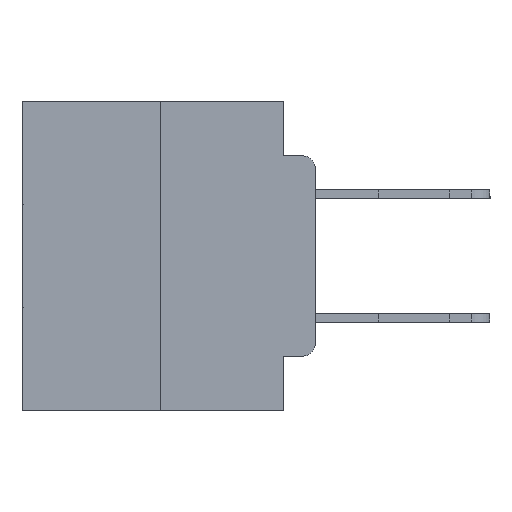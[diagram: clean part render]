
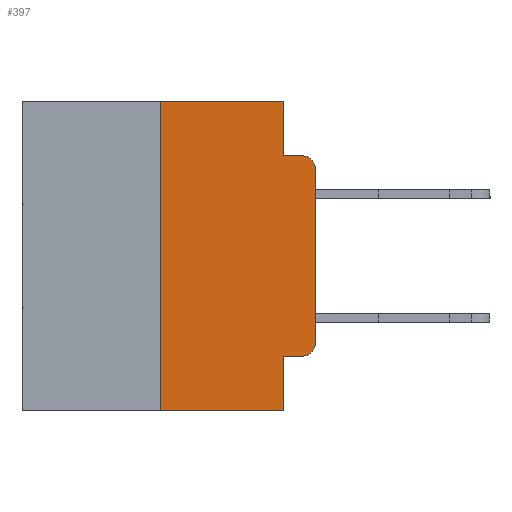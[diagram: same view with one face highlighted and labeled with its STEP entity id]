
A CAD part, left-side view. The second image highlights one B-rep face of the part: STEP entity #397.
In plain terms, the highlighted planar face has unit normal (-1, 0, 0).
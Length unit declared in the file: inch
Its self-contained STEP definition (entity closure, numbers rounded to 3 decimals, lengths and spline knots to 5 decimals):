
#229 = LINE ( 'NONE', #26358, #16529 ) ;
#397 = ADVANCED_FACE ( 'NONE', ( #26784 ), #27056, .F. ) ;
#853 = VERTEX_POINT ( 'NONE', #21630 ) ;
#1087 = VECTOR ( 'NONE', #23275, 39.37008 ) ;
#1859 = ORIENTED_EDGE ( 'NONE', *, *, #12511, .F. ) ;
#2058 = LINE ( 'NONE', #12790, #23794 ) ;
#2089 = CARTESIAN_POINT ( 'NONE',  ( 0., 0.051, 0. ) ) ;
#2174 = VERTEX_POINT ( 'NONE', #6560 ) ;
#2223 = ORIENTED_EDGE ( 'NONE', *, *, #10779, .T. ) ;
#2288 = LINE ( 'NONE', #14932, #2965 ) ;
#2649 = LINE ( 'NONE', #8467, #24348 ) ;
#2965 = VECTOR ( 'NONE', #25342, 39.37008 ) ;
#3467 = CARTESIAN_POINT ( 'NONE',  ( 0., 0.02, -0.1085 ) ) ;
#3753 = VECTOR ( 'NONE', #7286, 39.37008 ) ;
#4830 = CIRCLE ( 'NONE', #24839, 0.02 ) ;
#5434 = CARTESIAN_POINT ( 'NONE',  ( 0., 0., -0.1085 ) ) ;
#5666 = DIRECTION ( 'NONE',  ( 0., 0., -1. ) ) ;
#6070 = CARTESIAN_POINT ( 'NONE',  ( 0., 0.02, -0.0885 ) ) ;
#6560 = CARTESIAN_POINT ( 'NONE',  ( 0., 0.051, -0.5 ) ) ;
#7201 = CARTESIAN_POINT ( 'NONE',  ( 0., 0.051, -0.4115 ) ) ;
#7286 = DIRECTION ( 'NONE',  ( 0., -1., 0. ) ) ;
#7513 = VECTOR ( 'NONE', #23516, 39.37008 ) ;
#7628 = EDGE_CURVE ( 'NONE', #26926, #10000, #229, .T. ) ;
#7973 = EDGE_CURVE ( 'NONE', #22017, #853, #2288, .T. ) ;
#8064 = VECTOR ( 'NONE', #23064, 39.37008 ) ;
#8467 = CARTESIAN_POINT ( 'NONE',  ( 0., 0.051, 0. ) ) ;
#8608 = VERTEX_POINT ( 'NONE', #11317 ) ;
#9256 = AXIS2_PLACEMENT_3D ( 'NONE', #24442, #11910, #26522 ) ;
#9605 = DIRECTION ( 'NONE',  ( 0., 0., 1. ) ) ;
#10000 = VERTEX_POINT ( 'NONE', #5434 ) ;
#10397 = EDGE_CURVE ( 'NONE', #13606, #19159, #17350, .T. ) ;
#10779 = EDGE_CURVE ( 'NONE', #853, #26926, #12392, .T. ) ;
#10858 = ORIENTED_EDGE ( 'NONE', *, *, #18892, .F. ) ;
#10883 = CARTESIAN_POINT ( 'NONE',  ( 0., 0.051, 0. ) ) ;
#11314 = VERTEX_POINT ( 'NONE', #20192 ) ;
#11317 = CARTESIAN_POINT ( 'NONE',  ( 0., 0.25, 0. ) ) ;
#11460 = CARTESIAN_POINT ( 'NONE',  ( 0., 0.473, 0. ) ) ;
#11822 = ORIENTED_EDGE ( 'NONE', *, *, #10397, .F. ) ;
#11910 = DIRECTION ( 'NONE',  ( -1., 0., 0. ) ) ;
#12165 = ORIENTED_EDGE ( 'NONE', *, *, #7973, .T. ) ;
#12392 = CIRCLE ( 'NONE', #9256, 0.02 ) ;
#12511 = EDGE_CURVE ( 'NONE', #8608, #24337, #20532, .T. ) ;
#12790 = CARTESIAN_POINT ( 'NONE',  ( 0., 0.473, -0.5 ) ) ;
#13057 = LINE ( 'NONE', #10883, #7513 ) ;
#13606 = VERTEX_POINT ( 'NONE', #19401 ) ;
#13658 = CARTESIAN_POINT ( 'NONE',  ( 0., 0., -0.3915 ) ) ;
#14806 = DIRECTION ( 'NONE',  ( 0., 0., -1. ) ) ;
#14932 = CARTESIAN_POINT ( 'NONE',  ( 0., 0.051, -0.4115 ) ) ;
#14963 = CARTESIAN_POINT ( 'NONE',  ( 0., 0.051, -0.0885 ) ) ;
#16049 = EDGE_CURVE ( 'NONE', #24337, #13606, #13057, .T. ) ;
#16089 = ORIENTED_EDGE ( 'NONE', *, *, #7628, .T. ) ;
#16529 = VECTOR ( 'NONE', #9605, 39.37008 ) ;
#17106 = EDGE_CURVE ( 'NONE', #11314, #2174, #2058, .T. ) ;
#17350 = LINE ( 'NONE', #14963, #1087 ) ;
#17455 = EDGE_CURVE ( 'NONE', #10000, #19159, #4830, .T. ) ;
#18069 = CARTESIAN_POINT ( 'NONE',  ( 0., 0.473, 0. ) ) ;
#18087 = ORIENTED_EDGE ( 'NONE', *, *, #16049, .F. ) ;
#18202 = DIRECTION ( 'NONE',  ( -1., 0., 0. ) ) ;
#18892 = EDGE_CURVE ( 'NONE', #22017, #2174, #2649, .T. ) ;
#19154 = DIRECTION ( 'NONE',  ( 0., -1., 0. ) ) ;
#19159 = VERTEX_POINT ( 'NONE', #6070 ) ;
#19401 = CARTESIAN_POINT ( 'NONE',  ( 0., 0.051, -0.0885 ) ) ;
#19532 = AXIS2_PLACEMENT_3D ( 'NONE', #18069, #27087, #26939 ) ;
#20192 = CARTESIAN_POINT ( 'NONE',  ( 0., 0.25, -0.5 ) ) ;
#20532 = LINE ( 'NONE', #11460, #3753 ) ;
#20722 = ORIENTED_EDGE ( 'NONE', *, *, #23048, .F. ) ;
#21001 = CARTESIAN_POINT ( 'NONE',  ( 0., 0.25, 0. ) ) ;
#21630 = CARTESIAN_POINT ( 'NONE',  ( 0., 0.02, -0.4115 ) ) ;
#22017 = VERTEX_POINT ( 'NONE', #7201 ) ;
#22318 = ORIENTED_EDGE ( 'NONE', *, *, #17455, .T. ) ;
#23048 = EDGE_CURVE ( 'NONE', #11314, #8608, #24752, .T. ) ;
#23064 = DIRECTION ( 'NONE',  ( 0., 0., 1. ) ) ;
#23275 = DIRECTION ( 'NONE',  ( 0., -1., 0. ) ) ;
#23516 = DIRECTION ( 'NONE',  ( 0., 0., -1. ) ) ;
#23794 = VECTOR ( 'NONE', #19154, 39.37008 ) ;
#24337 = VERTEX_POINT ( 'NONE', #2089 ) ;
#24348 = VECTOR ( 'NONE', #14806, 39.37008 ) ;
#24442 = CARTESIAN_POINT ( 'NONE',  ( 0., 0.02, -0.3915 ) ) ;
#24752 = LINE ( 'NONE', #21001, #8064 ) ;
#24839 = AXIS2_PLACEMENT_3D ( 'NONE', #3467, #18202, #5666 ) ;
#25342 = DIRECTION ( 'NONE',  ( 0., -1., 0. ) ) ;
#26222 = ORIENTED_EDGE ( 'NONE', *, *, #17106, .T. ) ;
#26358 = CARTESIAN_POINT ( 'NONE',  ( 0., 0., 0. ) ) ;
#26522 = DIRECTION ( 'NONE',  ( 0., 0., -1. ) ) ;
#26614 = EDGE_LOOP ( 'NONE', ( #16089, #22318, #11822, #18087, #1859, #20722, #26222, #10858, #12165, #2223 ) ) ;
#26784 = FACE_OUTER_BOUND ( 'NONE', #26614, .T. ) ;
#26926 = VERTEX_POINT ( 'NONE', #13658 ) ;
#26939 = DIRECTION ( 'NONE',  ( 0., 0., -1. ) ) ;
#27056 = PLANE ( 'NONE',  #19532 ) ;
#27087 = DIRECTION ( 'NONE',  ( 1., 0., 0. ) ) ;
